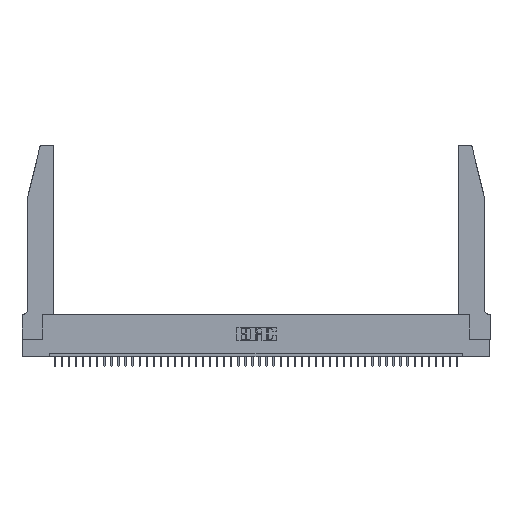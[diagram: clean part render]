
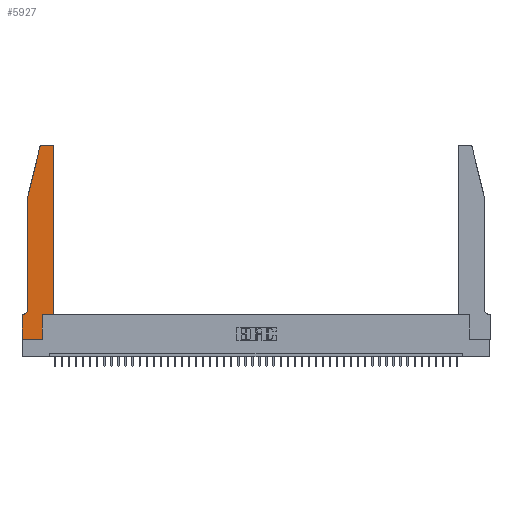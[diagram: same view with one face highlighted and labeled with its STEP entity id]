
A CAD part, top view. The second image highlights one B-rep face of the part: STEP entity #5927.
In plain terms, the highlighted planar face has unit normal (0, 0, 1).
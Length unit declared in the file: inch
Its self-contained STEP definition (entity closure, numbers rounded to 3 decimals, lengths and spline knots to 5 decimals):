
#603 = EDGE_CURVE ( 'NONE', #4234, #45382, #36778, .T. ) ;
#1009 = ORIENTED_EDGE ( 'NONE', *, *, #35822, .T. ) ;
#1043 = ORIENTED_EDGE ( 'NONE', *, *, #31957, .T. ) ;
#1157 = LINE ( 'NONE', #15451, #3447 ) ;
#1451 = CARTESIAN_POINT ( 'NONE',  ( 0.0755, 2., 0.37 ) ) ;
#1497 = EDGE_CURVE ( 'NONE', #40412, #24691, #44103, .T. ) ;
#2762 = DIRECTION ( 'NONE',  ( -1., 0., 0. ) ) ;
#3164 = CARTESIAN_POINT ( 'NONE',  ( 0., 0.35, 0.37 ) ) ;
#3447 = VECTOR ( 'NONE', #2762, 39.37008 ) ;
#3547 = VECTOR ( 'NONE', #10621, 39.37008 ) ;
#4234 = VERTEX_POINT ( 'NONE', #32972 ) ;
#4585 = CARTESIAN_POINT ( 'NONE',  ( 0.0755, 2., 0.37 ) ) ;
#5238 = ORIENTED_EDGE ( 'NONE', *, *, #32112, .T. ) ;
#5613 = EDGE_CURVE ( 'NONE', #28376, #22845, #46025, .T. ) ;
#5927 = ADVANCED_FACE ( 'NONE', ( #20810 ), #31355, .T. ) ;
#6019 = CARTESIAN_POINT ( 'NONE',  ( 0.4505, 2.72, 0.37 ) ) ;
#6440 = DIRECTION ( 'NONE',  ( 0., 1., 0. ) ) ;
#6661 = LINE ( 'NONE', #31303, #9215 ) ;
#7613 = VERTEX_POINT ( 'NONE', #3164 ) ;
#7782 = ORIENTED_EDGE ( 'NONE', *, *, #26873, .T. ) ;
#8821 = EDGE_CURVE ( 'NONE', #40652, #34649, #31948, .T. ) ;
#8939 = DIRECTION ( 'NONE',  ( -0.239, -0.971, 0. ) ) ;
#9017 = DIRECTION ( 'NONE',  ( 1., 0., 0. ) ) ;
#9215 = VECTOR ( 'NONE', #32228, 39.37008 ) ;
#9784 = EDGE_CURVE ( 'NONE', #26194, #33799, #34344, .T. ) ;
#9850 = CARTESIAN_POINT ( 'NONE',  ( 0.0755, 0.35, 0.37 ) ) ;
#10293 = DIRECTION ( 'NONE',  ( 0., -1., 0. ) ) ;
#10621 = DIRECTION ( 'NONE',  ( 0., -1., 0. ) ) ;
#11681 = DIRECTION ( 'NONE',  ( 1., 0., 0. ) ) ;
#13472 = VECTOR ( 'NONE', #8939, 39.37008 ) ;
#13923 = VECTOR ( 'NONE', #6440, 39.37008 ) ;
#15425 = ORIENTED_EDGE ( 'NONE', *, *, #8821, .T. ) ;
#15451 = CARTESIAN_POINT ( 'NONE',  ( 0.2605, 2.75, 0.37 ) ) ;
#15603 = VECTOR ( 'NONE', #9017, 39.37008 ) ;
#15785 = CARTESIAN_POINT ( 'NONE',  ( 0.4205, 2.75, 0.37 ) ) ;
#15912 = DIRECTION ( 'NONE',  ( 0., 0., 1. ) ) ;
#17859 = ORIENTED_EDGE ( 'NONE', *, *, #39812, .T. ) ;
#18401 = AXIS2_PLACEMENT_3D ( 'NONE', #28549, #46113, #39090 ) ;
#19290 = LINE ( 'NONE', #1451, #13472 ) ;
#19997 = EDGE_LOOP ( 'NONE', ( #5238, #31300, #27876, #15425, #17859, #1009, #1043, #37713, #36242, #34829, #7782, #43613 ) ) ;
#20744 = DIRECTION ( 'NONE',  ( -1., 0., 0. ) ) ;
#20810 = FACE_OUTER_BOUND ( 'NONE', #19997, .T. ) ;
#21675 = EDGE_CURVE ( 'NONE', #22845, #40652, #19290, .T. ) ;
#22708 = CARTESIAN_POINT ( 'NONE',  ( 0.4505, 0.35, 0.37 ) ) ;
#22842 = CARTESIAN_POINT ( 'NONE',  ( 0.4205, 2.72, 0.37 ) ) ;
#22845 = VERTEX_POINT ( 'NONE', #29164 ) ;
#24691 = VERTEX_POINT ( 'NONE', #15785 ) ;
#24775 = LINE ( 'NONE', #31324, #13923 ) ;
#24926 = CARTESIAN_POINT ( 'NONE',  ( 0.2865, 0.35, 0.37 ) ) ;
#26194 = VERTEX_POINT ( 'NONE', #24926 ) ;
#26873 = EDGE_CURVE ( 'NONE', #33799, #40412, #6661, .T. ) ;
#27876 = ORIENTED_EDGE ( 'NONE', *, *, #21675, .T. ) ;
#28150 = LINE ( 'NONE', #42437, #43869 ) ;
#28376 = VERTEX_POINT ( 'NONE', #34818 ) ;
#28549 = CARTESIAN_POINT ( 'NONE',  ( 0., 0.35, 0.37 ) ) ;
#29164 = CARTESIAN_POINT ( 'NONE',  ( 0.25487, 2.72718, 0.37 ) ) ;
#29875 = DIRECTION ( 'NONE',  ( 1., 0., 0. ) ) ;
#31300 = ORIENTED_EDGE ( 'NONE', *, *, #5613, .T. ) ;
#31303 = CARTESIAN_POINT ( 'NONE',  ( 0.4505, 0.35, 0.37 ) ) ;
#31324 = CARTESIAN_POINT ( 'NONE',  ( 0.2865, 0.35, 0.37 ) ) ;
#31355 = PLANE ( 'NONE',  #18401 ) ;
#31520 = CARTESIAN_POINT ( 'NONE',  ( 0.0055, 0.42, 0.37 ) ) ;
#31582 = VERTEX_POINT ( 'NONE', #36388 ) ;
#31948 = LINE ( 'NONE', #42756, #3547 ) ;
#31957 = EDGE_CURVE ( 'NONE', #7613, #4234, #28150, .T. ) ;
#32112 = EDGE_CURVE ( 'NONE', #24691, #28376, #1157, .T. ) ;
#32228 = DIRECTION ( 'NONE',  ( 0., 1., 0. ) ) ;
#32650 = CARTESIAN_POINT ( 'NONE',  ( 0.0755, 0.42, 0.37 ) ) ;
#32732 = EDGE_CURVE ( 'NONE', #45382, #26194, #24775, .T. ) ;
#32972 = CARTESIAN_POINT ( 'NONE',  ( 0., 0., 0.37 ) ) ;
#33415 = CARTESIAN_POINT ( 'NONE',  ( 0.4505, 0.35, 0.37 ) ) ;
#33799 = VERTEX_POINT ( 'NONE', #22708 ) ;
#34344 = LINE ( 'NONE', #33415, #15603 ) ;
#34649 = VERTEX_POINT ( 'NONE', #32650 ) ;
#34818 = CARTESIAN_POINT ( 'NONE',  ( 0.284, 2.75, 0.37 ) ) ;
#34829 = ORIENTED_EDGE ( 'NONE', *, *, #9784, .T. ) ;
#35489 = DIRECTION ( 'NONE',  ( 0., 0., -1. ) ) ;
#35822 = EDGE_CURVE ( 'NONE', #31582, #7613, #41293, .T. ) ;
#36242 = ORIENTED_EDGE ( 'NONE', *, *, #32732, .T. ) ;
#36388 = CARTESIAN_POINT ( 'NONE',  ( 0.0055, 0.35, 0.37 ) ) ;
#36722 = AXIS2_PLACEMENT_3D ( 'NONE', #31520, #35489, #20744 ) ;
#36778 = LINE ( 'NONE', #43360, #39527 ) ;
#37455 = CIRCLE ( 'NONE', #36722, 0.07 ) ;
#37713 = ORIENTED_EDGE ( 'NONE', *, *, #603, .T. ) ;
#37770 = DIRECTION ( 'NONE',  ( -1., 0., 0. ) ) ;
#38493 = CARTESIAN_POINT ( 'NONE',  ( 0.2865, 0., 0.37 ) ) ;
#39090 = DIRECTION ( 'NONE',  ( 1., 0., 0. ) ) ;
#39527 = VECTOR ( 'NONE', #11681, 39.37008 ) ;
#39812 = EDGE_CURVE ( 'NONE', #34649, #31582, #37455, .T. ) ;
#40412 = VERTEX_POINT ( 'NONE', #6019 ) ;
#40652 = VERTEX_POINT ( 'NONE', #4585 ) ;
#41066 = AXIS2_PLACEMENT_3D ( 'NONE', #22842, #44408, #29875 ) ;
#41293 = LINE ( 'NONE', #9850, #41716 ) ;
#41716 = VECTOR ( 'NONE', #37770, 39.37008 ) ;
#42437 = CARTESIAN_POINT ( 'NONE',  ( 0., 0., 0.37 ) ) ;
#42756 = CARTESIAN_POINT ( 'NONE',  ( 0.0755, 2., 0.37 ) ) ;
#43063 = AXIS2_PLACEMENT_3D ( 'NONE', #44047, #15912, #43595 ) ;
#43360 = CARTESIAN_POINT ( 'NONE',  ( 0., 0., 0.37 ) ) ;
#43595 = DIRECTION ( 'NONE',  ( 1., 0., 0. ) ) ;
#43613 = ORIENTED_EDGE ( 'NONE', *, *, #1497, .T. ) ;
#43869 = VECTOR ( 'NONE', #10293, 39.37008 ) ;
#44047 = CARTESIAN_POINT ( 'NONE',  ( 0.284, 2.72, 0.37 ) ) ;
#44103 = CIRCLE ( 'NONE', #41066, 0.03 ) ;
#44408 = DIRECTION ( 'NONE',  ( 0., 0., 1. ) ) ;
#45382 = VERTEX_POINT ( 'NONE', #38493 ) ;
#46025 = CIRCLE ( 'NONE', #43063, 0.03 ) ;
#46113 = DIRECTION ( 'NONE',  ( 0., 0., 1. ) ) ;
